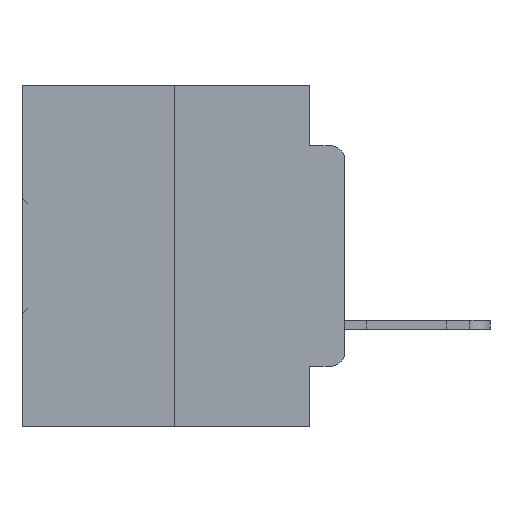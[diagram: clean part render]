
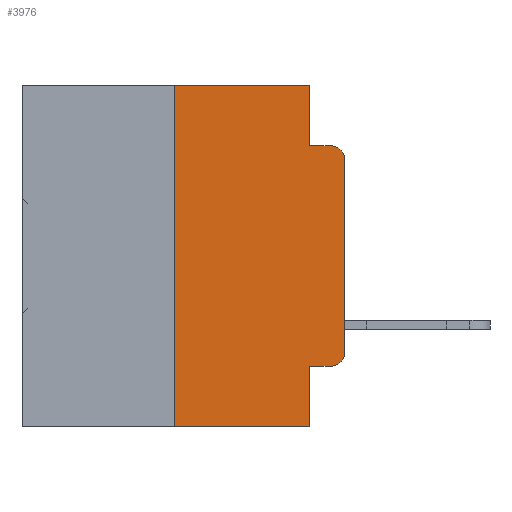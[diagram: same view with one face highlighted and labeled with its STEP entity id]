
A CAD part, left-side view. The second image highlights one B-rep face of the part: STEP entity #3976.
In plain terms, the highlighted planar face has unit normal (-1, 0, 0).
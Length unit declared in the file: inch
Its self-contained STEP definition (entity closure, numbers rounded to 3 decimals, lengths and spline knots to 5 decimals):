
#309 = LINE ( 'NONE', #21165, #14956 ) ;
#1665 = VECTOR ( 'NONE', #22682, 39.37008 ) ;
#1772 = EDGE_CURVE ( 'NONE', #21609, #14376, #34424, .T. ) ;
#2410 = DIRECTION ( 'NONE',  ( -1., 0., 0. ) ) ;
#2987 = CARTESIAN_POINT ( 'NONE',  ( 0., 0.02, -0.3915 ) ) ;
#3062 = ORIENTED_EDGE ( 'NONE', *, *, #3777, .F. ) ;
#3627 = VECTOR ( 'NONE', #15730, 39.37008 ) ;
#3777 = EDGE_CURVE ( 'NONE', #14086, #23462, #29972, .T. ) ;
#3976 = ADVANCED_FACE ( 'NONE', ( #17419 ), #23619, .F. ) ;
#4007 = CIRCLE ( 'NONE', #16503, 0.02 ) ;
#4617 = DIRECTION ( 'NONE',  ( 0., -1., 0. ) ) ;
#5194 = VERTEX_POINT ( 'NONE', #10661 ) ;
#6078 = DIRECTION ( 'NONE',  ( 0., 0., -1. ) ) ;
#7749 = CARTESIAN_POINT ( 'NONE',  ( 0., 0., -0.1085 ) ) ;
#7860 = ORIENTED_EDGE ( 'NONE', *, *, #26105, .T. ) ;
#7965 = VERTEX_POINT ( 'NONE', #33356 ) ;
#9451 = VERTEX_POINT ( 'NONE', #7749 ) ;
#10661 = CARTESIAN_POINT ( 'NONE',  ( 0., 0., -0.3915 ) ) ;
#11384 = VERTEX_POINT ( 'NONE', #31674 ) ;
#11931 = EDGE_CURVE ( 'NONE', #14086, #14376, #31312, .T. ) ;
#12170 = CARTESIAN_POINT ( 'NONE',  ( 0., 0.051, -0.4115 ) ) ;
#12472 = CARTESIAN_POINT ( 'NONE',  ( 0., 0.25, 0. ) ) ;
#12799 = DIRECTION ( 'NONE',  ( 0., 0., -1. ) ) ;
#13022 = EDGE_LOOP ( 'NONE', ( #22945, #7860, #28603, #24339, #28685, #3062, #23287, #17834, #18280, #29991 ) ) ;
#13105 = CARTESIAN_POINT ( 'NONE',  ( 0., 0.473, 0. ) ) ;
#13392 = VECTOR ( 'NONE', #15818, 39.37008 ) ;
#14086 = VERTEX_POINT ( 'NONE', #22971 ) ;
#14376 = VERTEX_POINT ( 'NONE', #15281 ) ;
#14463 = CARTESIAN_POINT ( 'NONE',  ( 0., 0.02, -0.0885 ) ) ;
#14956 = VECTOR ( 'NONE', #23853, 39.37008 ) ;
#15149 = CARTESIAN_POINT ( 'NONE',  ( 0., 0.051, 0. ) ) ;
#15281 = CARTESIAN_POINT ( 'NONE',  ( 0., 0.051, -0.5 ) ) ;
#15373 = EDGE_CURVE ( 'NONE', #21781, #11384, #25031, .T. ) ;
#15730 = DIRECTION ( 'NONE',  ( 0., 0., -1. ) ) ;
#15818 = DIRECTION ( 'NONE',  ( 0., -1., 0. ) ) ;
#16503 = AXIS2_PLACEMENT_3D ( 'NONE', #19415, #2410, #22156 ) ;
#17059 = DIRECTION ( 'NONE',  ( 0., -1., 0. ) ) ;
#17111 = CARTESIAN_POINT ( 'NONE',  ( 0., 0.473, -0.5 ) ) ;
#17122 = CIRCLE ( 'NONE', #21887, 0.02 ) ;
#17419 = FACE_OUTER_BOUND ( 'NONE', #13022, .T. ) ;
#17834 = ORIENTED_EDGE ( 'NONE', *, *, #1772, .F. ) ;
#18280 = ORIENTED_EDGE ( 'NONE', *, *, #25042, .T. ) ;
#19415 = CARTESIAN_POINT ( 'NONE',  ( 0., 0.02, -0.1085 ) ) ;
#19683 = CARTESIAN_POINT ( 'NONE',  ( 0., 0.051, 0. ) ) ;
#21165 = CARTESIAN_POINT ( 'NONE',  ( 0., 0.051, -0.4115 ) ) ;
#21246 = LINE ( 'NONE', #25774, #34355 ) ;
#21452 = LINE ( 'NONE', #13105, #13392 ) ;
#21609 = VERTEX_POINT ( 'NONE', #12170 ) ;
#21781 = VERTEX_POINT ( 'NONE', #26376 ) ;
#21887 = AXIS2_PLACEMENT_3D ( 'NONE', #2987, #22684, #6078 ) ;
#22156 = DIRECTION ( 'NONE',  ( 0., 0., -1. ) ) ;
#22682 = DIRECTION ( 'NONE',  ( 0., 0., 1. ) ) ;
#22684 = DIRECTION ( 'NONE',  ( -1., 0., 0. ) ) ;
#22945 = ORIENTED_EDGE ( 'NONE', *, *, #34100, .T. ) ;
#22971 = CARTESIAN_POINT ( 'NONE',  ( 0., 0.25, -0.5 ) ) ;
#23272 = EDGE_CURVE ( 'NONE', #7965, #5194, #17122, .T. ) ;
#23287 = ORIENTED_EDGE ( 'NONE', *, *, #11931, .T. ) ;
#23462 = VERTEX_POINT ( 'NONE', #12472 ) ;
#23590 = DIRECTION ( 'NONE',  ( 1., 0., 0. ) ) ;
#23619 = PLANE ( 'NONE',  #29066 ) ;
#23853 = DIRECTION ( 'NONE',  ( 0., -1., 0. ) ) ;
#24014 = CARTESIAN_POINT ( 'NONE',  ( 0., 0.051, -0.0885 ) ) ;
#24289 = DIRECTION ( 'NONE',  ( 0., 0., -1. ) ) ;
#24339 = ORIENTED_EDGE ( 'NONE', *, *, #15373, .F. ) ;
#24408 = EDGE_CURVE ( 'NONE', #11384, #32665, #25444, .T. ) ;
#25031 = LINE ( 'NONE', #15149, #3627 ) ;
#25042 = EDGE_CURVE ( 'NONE', #21609, #7965, #309, .T. ) ;
#25137 = CARTESIAN_POINT ( 'NONE',  ( 0., 0.25, 0. ) ) ;
#25444 = LINE ( 'NONE', #24014, #31193 ) ;
#25774 = CARTESIAN_POINT ( 'NONE',  ( 0., 0., 0. ) ) ;
#26105 = EDGE_CURVE ( 'NONE', #9451, #32665, #4007, .T. ) ;
#26376 = CARTESIAN_POINT ( 'NONE',  ( 0., 0.051, 0. ) ) ;
#26650 = VECTOR ( 'NONE', #24289, 39.37008 ) ;
#28298 = DIRECTION ( 'NONE',  ( 0., 0., 1. ) ) ;
#28603 = ORIENTED_EDGE ( 'NONE', *, *, #24408, .F. ) ;
#28685 = ORIENTED_EDGE ( 'NONE', *, *, #30464, .F. ) ;
#29066 = AXIS2_PLACEMENT_3D ( 'NONE', #30916, #23590, #12799 ) ;
#29972 = LINE ( 'NONE', #25137, #1665 ) ;
#29991 = ORIENTED_EDGE ( 'NONE', *, *, #23272, .T. ) ;
#30464 = EDGE_CURVE ( 'NONE', #23462, #21781, #21452, .T. ) ;
#30916 = CARTESIAN_POINT ( 'NONE',  ( 0., 0.473, 0. ) ) ;
#31193 = VECTOR ( 'NONE', #4617, 39.37008 ) ;
#31312 = LINE ( 'NONE', #17111, #32022 ) ;
#31674 = CARTESIAN_POINT ( 'NONE',  ( 0., 0.051, -0.0885 ) ) ;
#32022 = VECTOR ( 'NONE', #17059, 39.37008 ) ;
#32665 = VERTEX_POINT ( 'NONE', #14463 ) ;
#33356 = CARTESIAN_POINT ( 'NONE',  ( 0., 0.02, -0.4115 ) ) ;
#34100 = EDGE_CURVE ( 'NONE', #5194, #9451, #21246, .T. ) ;
#34355 = VECTOR ( 'NONE', #28298, 39.37008 ) ;
#34424 = LINE ( 'NONE', #19683, #26650 ) ;
